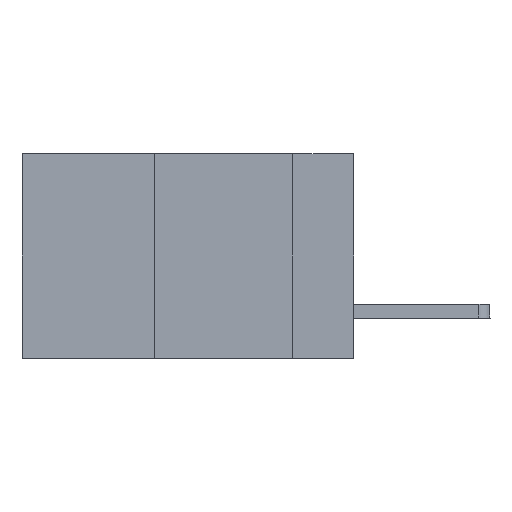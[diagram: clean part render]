
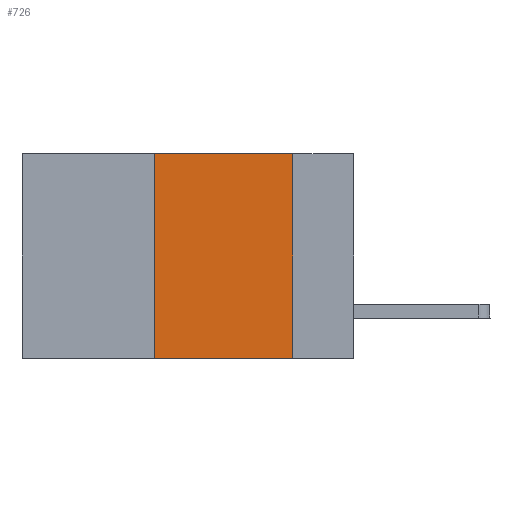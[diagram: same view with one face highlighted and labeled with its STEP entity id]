
A CAD part, left-side view. The second image highlights one B-rep face of the part: STEP entity #726.
In plain terms, the highlighted planar face has unit normal (-1, 0, 0).
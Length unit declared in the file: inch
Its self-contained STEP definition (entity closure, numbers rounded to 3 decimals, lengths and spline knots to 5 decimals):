
#657 = VECTOR ( 'NONE', #5502, 39.37008 ) ;
#726 = ADVANCED_FACE ( 'NONE', ( #10259 ), #10180, .F. ) ;
#1882 = ORIENTED_EDGE ( 'NONE', *, *, #10313, .F. ) ;
#2356 = CARTESIAN_POINT ( 'NONE',  ( 0., 0.11, -0.37 ) ) ;
#3062 = LINE ( 'NONE', #5752, #11397 ) ;
#3374 = LINE ( 'NONE', #11536, #657 ) ;
#3686 = ORIENTED_EDGE ( 'NONE', *, *, #11783, .F. ) ;
#3838 = VECTOR ( 'NONE', #5268, 39.37008 ) ;
#4260 = AXIS2_PLACEMENT_3D ( 'NONE', #8261, #5330, #6278 ) ;
#4462 = VECTOR ( 'NONE', #9925, 39.37008 ) ;
#4773 = LINE ( 'NONE', #11308, #3838 ) ;
#5070 = CARTESIAN_POINT ( 'NONE',  ( 0., 0.6, 0. ) ) ;
#5087 = EDGE_CURVE ( 'NONE', #8944, #11888, #3062, .T. ) ;
#5268 = DIRECTION ( 'NONE',  ( 0., 0., -1. ) ) ;
#5330 = DIRECTION ( 'NONE',  ( 1., 0., 0. ) ) ;
#5502 = DIRECTION ( 'NONE',  ( 0., 0., 1. ) ) ;
#5752 = CARTESIAN_POINT ( 'NONE',  ( 0., 0.6, -0.37 ) ) ;
#5907 = VERTEX_POINT ( 'NONE', #11962 ) ;
#5975 = VERTEX_POINT ( 'NONE', #8852 ) ;
#6278 = DIRECTION ( 'NONE',  ( 0., 0., -1. ) ) ;
#6510 = EDGE_LOOP ( 'NONE', ( #3686, #8141, #1882, #11003 ) ) ;
#8141 = ORIENTED_EDGE ( 'NONE', *, *, #10465, .F. ) ;
#8261 = CARTESIAN_POINT ( 'NONE',  ( 0., 0.6, 0. ) ) ;
#8852 = CARTESIAN_POINT ( 'NONE',  ( 0., 0.11, 0. ) ) ;
#8944 = VERTEX_POINT ( 'NONE', #11040 ) ;
#9925 = DIRECTION ( 'NONE',  ( 0., -1., 0. ) ) ;
#10180 = PLANE ( 'NONE',  #4260 ) ;
#10259 = FACE_OUTER_BOUND ( 'NONE', #6510, .T. ) ;
#10313 = EDGE_CURVE ( 'NONE', #8944, #5907, #3374, .T. ) ;
#10465 = EDGE_CURVE ( 'NONE', #5907, #5975, #12352, .T. ) ;
#11003 = ORIENTED_EDGE ( 'NONE', *, *, #5087, .T. ) ;
#11040 = CARTESIAN_POINT ( 'NONE',  ( 0., 0.36, -0.37 ) ) ;
#11308 = CARTESIAN_POINT ( 'NONE',  ( 0., 0.11, 0. ) ) ;
#11397 = VECTOR ( 'NONE', #11913, 39.37008 ) ;
#11536 = CARTESIAN_POINT ( 'NONE',  ( 0., 0.36, 0. ) ) ;
#11783 = EDGE_CURVE ( 'NONE', #5975, #11888, #4773, .T. ) ;
#11888 = VERTEX_POINT ( 'NONE', #2356 ) ;
#11913 = DIRECTION ( 'NONE',  ( 0., -1., 0. ) ) ;
#11962 = CARTESIAN_POINT ( 'NONE',  ( 0., 0.36, 0. ) ) ;
#12352 = LINE ( 'NONE', #5070, #4462 ) ;
